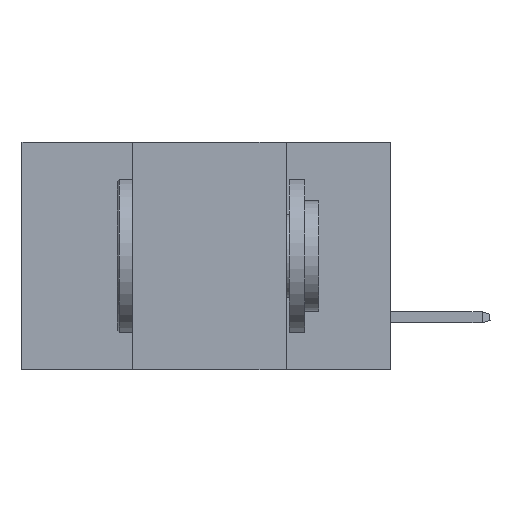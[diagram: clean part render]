
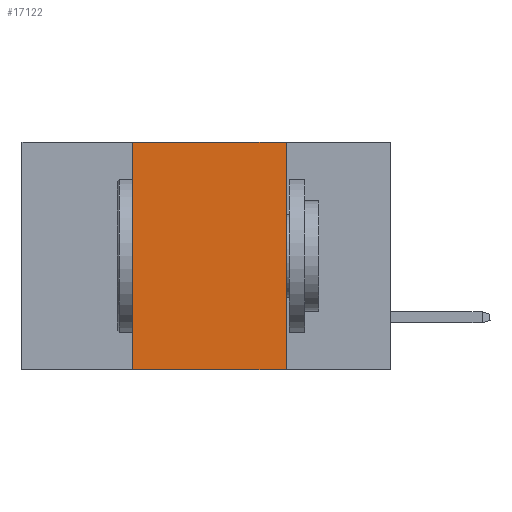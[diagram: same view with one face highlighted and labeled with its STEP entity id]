
A CAD part, left-side view. The second image highlights one B-rep face of the part: STEP entity #17122.
In plain terms, the highlighted planar face has unit normal (-1, 0, 0).
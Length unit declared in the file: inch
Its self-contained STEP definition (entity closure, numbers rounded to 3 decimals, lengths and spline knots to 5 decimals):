
#520 = VECTOR ( 'NONE', #766, 39.37008 ) ;
#766 = DIRECTION ( 'NONE',  ( 0., 0., 1. ) ) ;
#824 = ORIENTED_EDGE ( 'NONE', *, *, #6721, .F. ) ;
#1144 = CARTESIAN_POINT ( 'NONE',  ( 0., 0.6, 0. ) ) ;
#1817 = ORIENTED_EDGE ( 'NONE', *, *, #22951, .T. ) ;
#2442 = CARTESIAN_POINT ( 'NONE',  ( 0., 0.42, 0. ) ) ;
#3152 = LINE ( 'NONE', #8204, #13355 ) ;
#3233 = DIRECTION ( 'NONE',  ( 0., 0., -1. ) ) ;
#3806 = AXIS2_PLACEMENT_3D ( 'NONE', #1144, #15460, #3233 ) ;
#4028 = VERTEX_POINT ( 'NONE', #2442 ) ;
#4283 = VERTEX_POINT ( 'NONE', #13862 ) ;
#6087 = LINE ( 'NONE', #19034, #520 ) ;
#6721 = EDGE_CURVE ( 'NONE', #4028, #9755, #3152, .T. ) ;
#6897 = VECTOR ( 'NONE', #19338, 39.37008 ) ;
#7778 = VECTOR ( 'NONE', #17102, 39.37008 ) ;
#7879 = VERTEX_POINT ( 'NONE', #24000 ) ;
#8204 = CARTESIAN_POINT ( 'NONE',  ( 0., 0.6, 0. ) ) ;
#9132 = FACE_OUTER_BOUND ( 'NONE', #24994, .T. ) ;
#9755 = VERTEX_POINT ( 'NONE', #13337 ) ;
#11754 = ORIENTED_EDGE ( 'NONE', *, *, #23960, .F. ) ;
#13337 = CARTESIAN_POINT ( 'NONE',  ( 0., 0.17, 0. ) ) ;
#13355 = VECTOR ( 'NONE', #22434, 39.37008 ) ;
#13862 = CARTESIAN_POINT ( 'NONE',  ( 0., 0.17, -0.37 ) ) ;
#15037 = CARTESIAN_POINT ( 'NONE',  ( 0., 0.17, 0. ) ) ;
#15130 = EDGE_CURVE ( 'NONE', #7879, #4028, #6087, .T. ) ;
#15376 = PLANE ( 'NONE',  #3806 ) ;
#15460 = DIRECTION ( 'NONE',  ( 1., 0., 0. ) ) ;
#15909 = ORIENTED_EDGE ( 'NONE', *, *, #15130, .F. ) ;
#17102 = DIRECTION ( 'NONE',  ( 0., 0., -1. ) ) ;
#17122 = ADVANCED_FACE ( 'NONE', ( #9132 ), #15376, .F. ) ;
#17289 = CARTESIAN_POINT ( 'NONE',  ( 0., 0.6, -0.37 ) ) ;
#17692 = LINE ( 'NONE', #17289, #6897 ) ;
#19034 = CARTESIAN_POINT ( 'NONE',  ( 0., 0.42, 0. ) ) ;
#19338 = DIRECTION ( 'NONE',  ( 0., -1., 0. ) ) ;
#22434 = DIRECTION ( 'NONE',  ( 0., -1., 0. ) ) ;
#22951 = EDGE_CURVE ( 'NONE', #7879, #4283, #17692, .T. ) ;
#23913 = LINE ( 'NONE', #15037, #7778 ) ;
#23960 = EDGE_CURVE ( 'NONE', #9755, #4283, #23913, .T. ) ;
#24000 = CARTESIAN_POINT ( 'NONE',  ( 0., 0.42, -0.37 ) ) ;
#24994 = EDGE_LOOP ( 'NONE', ( #11754, #824, #15909, #1817 ) ) ;
